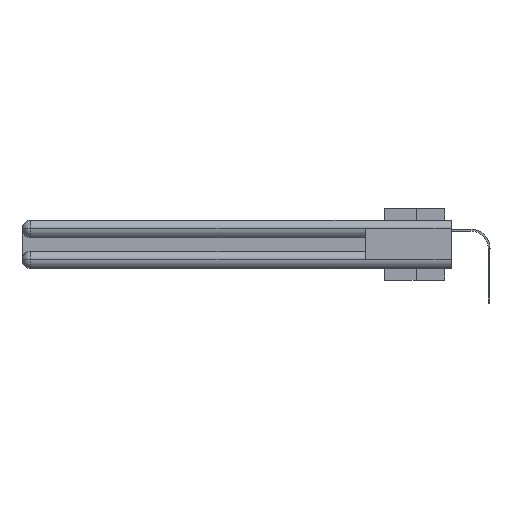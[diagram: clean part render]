
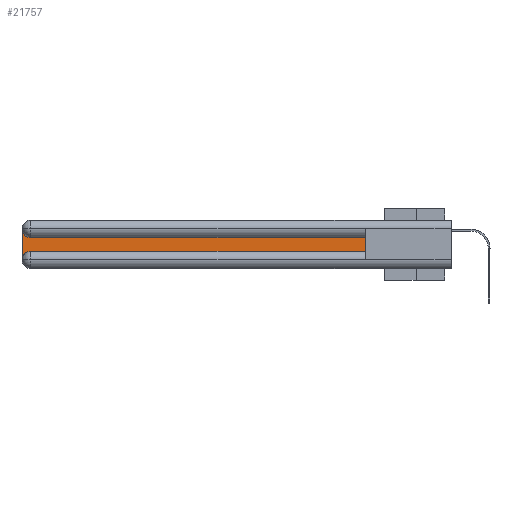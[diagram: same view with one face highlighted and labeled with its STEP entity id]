
A CAD part, left-side view. The second image highlights one B-rep face of the part: STEP entity #21757.
In plain terms, the highlighted planar face has unit normal (-1, 0, 0).
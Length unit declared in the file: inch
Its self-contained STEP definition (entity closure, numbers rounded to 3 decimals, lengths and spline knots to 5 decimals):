
#438 = ORIENTED_EDGE ( 'NONE', *, *, #23695, .T. ) ;
#2860 = CARTESIAN_POINT ( 'NONE',  ( 0.075, 2.94, -0.0625 ) ) ;
#3007 = DIRECTION ( 'NONE',  ( 0., 0., 1. ) ) ;
#3609 = DIRECTION ( 'NONE',  ( 1., 0., 0. ) ) ;
#4125 = VERTEX_POINT ( 'NONE', #24517 ) ;
#4468 = CARTESIAN_POINT ( 'NONE',  ( 0.075, 2.94, -0.2775 ) ) ;
#4970 = DIRECTION ( 'NONE',  ( 0., 1., 0. ) ) ;
#5007 = AXIS2_PLACEMENT_3D ( 'NONE', #4468, #13725, #22971 ) ;
#5488 = ORIENTED_EDGE ( 'NONE', *, *, #21924, .T. ) ;
#7691 = DIRECTION ( 'NONE',  ( 1., 0., 0. ) ) ;
#8464 = EDGE_CURVE ( 'NONE', #8648, #10025, #11984, .T. ) ;
#8648 = VERTEX_POINT ( 'NONE', #26492 ) ;
#9618 = LINE ( 'NONE', #18902, #29722 ) ;
#10025 = VERTEX_POINT ( 'NONE', #16128 ) ;
#10178 = VECTOR ( 'NONE', #4970, 39.37008 ) ;
#10561 = EDGE_CURVE ( 'NONE', #21005, #4125, #23758, .T. ) ;
#11399 = EDGE_CURVE ( 'NONE', #17068, #29346, #15682, .T. ) ;
#11984 = CIRCLE ( 'NONE', #15876, 0.06 ) ;
#12269 = VECTOR ( 'NONE', #3007, 39.37008 ) ;
#13725 = DIRECTION ( 'NONE',  ( 1., 0., 0. ) ) ;
#15414 = CARTESIAN_POINT ( 'NONE',  ( 0.075, 3., -0.1225 ) ) ;
#15682 = CIRCLE ( 'NONE', #5007, 0.06 ) ;
#15876 = AXIS2_PLACEMENT_3D ( 'NONE', #2860, #7691, #25749 ) ;
#16128 = CARTESIAN_POINT ( 'NONE',  ( 0.075, 3., -0.0625 ) ) ;
#16353 = LINE ( 'NONE', #21065, #10178 ) ;
#17068 = VERTEX_POINT ( 'NONE', #22143 ) ;
#17113 = CARTESIAN_POINT ( 'NONE',  ( 0.075, 2.94, -0.2175 ) ) ;
#17387 = PLANE ( 'NONE',  #22306 ) ;
#17839 = ORIENTED_EDGE ( 'NONE', *, *, #8464, .T. ) ;
#17923 = LINE ( 'NONE', #25043, #27189 ) ;
#18902 = CARTESIAN_POINT ( 'NONE',  ( 0.075, 3., -0.2175 ) ) ;
#18917 = CARTESIAN_POINT ( 'NONE',  ( 0.075, 0.6, -0.2175 ) ) ;
#20255 = ORIENTED_EDGE ( 'NONE', *, *, #10561, .T. ) ;
#20347 = DIRECTION ( 'NONE',  ( 0., -1., 0. ) ) ;
#21005 = VERTEX_POINT ( 'NONE', #25319 ) ;
#21043 = EDGE_LOOP ( 'NONE', ( #5488, #17839, #438, #27915, #29706, #20255 ) ) ;
#21065 = CARTESIAN_POINT ( 'NONE',  ( 0.075, 0.6, -0.1225 ) ) ;
#21757 = ADVANCED_FACE ( 'NONE', ( #26916 ), #17387, .F. ) ;
#21924 = EDGE_CURVE ( 'NONE', #4125, #8648, #16353, .T. ) ;
#22143 = CARTESIAN_POINT ( 'NONE',  ( 0.075, 3., -0.2775 ) ) ;
#22306 = AXIS2_PLACEMENT_3D ( 'NONE', #15414, #3609, #27071 ) ;
#22971 = DIRECTION ( 'NONE',  ( 0., 0., -1. ) ) ;
#23695 = EDGE_CURVE ( 'NONE', #10025, #17068, #9618, .T. ) ;
#23758 = LINE ( 'NONE', #18917, #12269 ) ;
#24517 = CARTESIAN_POINT ( 'NONE',  ( 0.075, 0.6, -0.1225 ) ) ;
#25043 = CARTESIAN_POINT ( 'NONE',  ( 0.075, 0.6, -0.2175 ) ) ;
#25319 = CARTESIAN_POINT ( 'NONE',  ( 0.075, 0.6, -0.2175 ) ) ;
#25749 = DIRECTION ( 'NONE',  ( 0., 0., -1. ) ) ;
#26492 = CARTESIAN_POINT ( 'NONE',  ( 0.075, 2.94, -0.1225 ) ) ;
#26916 = FACE_OUTER_BOUND ( 'NONE', #21043, .T. ) ;
#27071 = DIRECTION ( 'NONE',  ( 0., 0., -1. ) ) ;
#27189 = VECTOR ( 'NONE', #20347, 39.37008 ) ;
#27915 = ORIENTED_EDGE ( 'NONE', *, *, #11399, .T. ) ;
#28124 = DIRECTION ( 'NONE',  ( 0., 0., -1. ) ) ;
#29346 = VERTEX_POINT ( 'NONE', #17113 ) ;
#29706 = ORIENTED_EDGE ( 'NONE', *, *, #29951, .T. ) ;
#29722 = VECTOR ( 'NONE', #28124, 39.37008 ) ;
#29951 = EDGE_CURVE ( 'NONE', #29346, #21005, #17923, .T. ) ;
